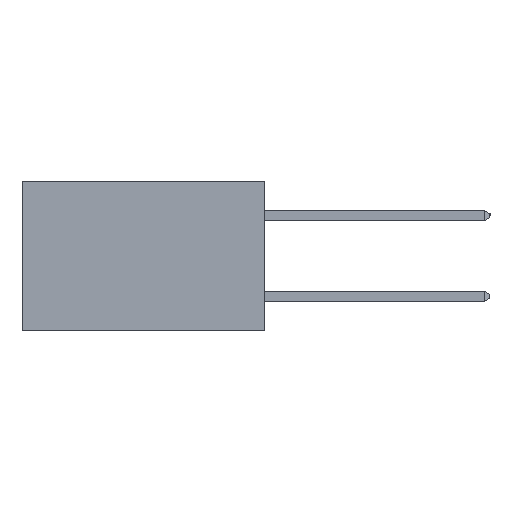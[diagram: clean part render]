
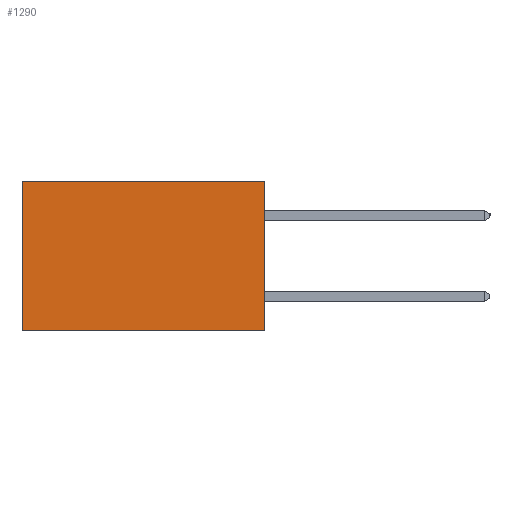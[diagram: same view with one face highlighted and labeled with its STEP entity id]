
A CAD part, left-side view. The second image highlights one B-rep face of the part: STEP entity #1290.
In plain terms, the highlighted planar face has unit normal (-1, 0, 0).
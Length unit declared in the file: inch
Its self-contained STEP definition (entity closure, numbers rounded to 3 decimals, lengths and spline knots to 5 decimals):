
#563 = VECTOR ( 'NONE', #10649, 39.37008 ) ;
#1081 = DIRECTION ( 'NONE',  ( 0., 0., -1. ) ) ;
#1290 = ADVANCED_FACE ( 'NONE', ( #22207 ), #18647, .F. ) ;
#1371 = EDGE_CURVE ( 'NONE', #7514, #8529, #21273, .T. ) ;
#1416 = EDGE_CURVE ( 'NONE', #7514, #10530, #5562, .T. ) ;
#2124 = VECTOR ( 'NONE', #17608, 39.37008 ) ;
#2860 = AXIS2_PLACEMENT_3D ( 'NONE', #22553, #16828, #1081 ) ;
#3380 = DIRECTION ( 'NONE',  ( 0., 0., -1. ) ) ;
#3419 = VERTEX_POINT ( 'NONE', #10369 ) ;
#4816 = LINE ( 'NONE', #8275, #10341 ) ;
#5429 = CARTESIAN_POINT ( 'NONE',  ( 0.2615, 0.6, 0. ) ) ;
#5562 = LINE ( 'NONE', #19330, #17175 ) ;
#7514 = VERTEX_POINT ( 'NONE', #19596 ) ;
#8130 = ORIENTED_EDGE ( 'NONE', *, *, #1371, .T. ) ;
#8205 = ORIENTED_EDGE ( 'NONE', *, *, #1416, .F. ) ;
#8275 = CARTESIAN_POINT ( 'NONE',  ( 0.2615, 0., -0.37 ) ) ;
#8529 = VERTEX_POINT ( 'NONE', #5429 ) ;
#10341 = VECTOR ( 'NONE', #17330, 39.37008 ) ;
#10369 = CARTESIAN_POINT ( 'NONE',  ( 0.2615, 0.6, -0.37 ) ) ;
#10431 = LINE ( 'NONE', #14105, #563 ) ;
#10530 = VERTEX_POINT ( 'NONE', #11378 ) ;
#10649 = DIRECTION ( 'NONE',  ( 0., 0., -1. ) ) ;
#10727 = EDGE_CURVE ( 'NONE', #10530, #3419, #4816, .T. ) ;
#11378 = CARTESIAN_POINT ( 'NONE',  ( 0.2615, 0., -0.37 ) ) ;
#12120 = CARTESIAN_POINT ( 'NONE',  ( 0.2615, 0., 0. ) ) ;
#14105 = CARTESIAN_POINT ( 'NONE',  ( 0.2615, 0.6, -0.37 ) ) ;
#15984 = ORIENTED_EDGE ( 'NONE', *, *, #17783, .T. ) ;
#16383 = EDGE_LOOP ( 'NONE', ( #15984, #22010, #8205, #8130 ) ) ;
#16828 = DIRECTION ( 'NONE',  ( 1., 0., 0. ) ) ;
#17175 = VECTOR ( 'NONE', #3380, 39.37008 ) ;
#17330 = DIRECTION ( 'NONE',  ( 0., 1., 0. ) ) ;
#17608 = DIRECTION ( 'NONE',  ( 0., 1., 0. ) ) ;
#17783 = EDGE_CURVE ( 'NONE', #8529, #3419, #10431, .T. ) ;
#18647 = PLANE ( 'NONE',  #2860 ) ;
#19330 = CARTESIAN_POINT ( 'NONE',  ( 0.2615, 0., -0.37 ) ) ;
#19596 = CARTESIAN_POINT ( 'NONE',  ( 0.2615, 0., 0. ) ) ;
#21273 = LINE ( 'NONE', #12120, #2124 ) ;
#22010 = ORIENTED_EDGE ( 'NONE', *, *, #10727, .F. ) ;
#22207 = FACE_OUTER_BOUND ( 'NONE', #16383, .T. ) ;
#22553 = CARTESIAN_POINT ( 'NONE',  ( 0.2615, 0., -0.37 ) ) ;
